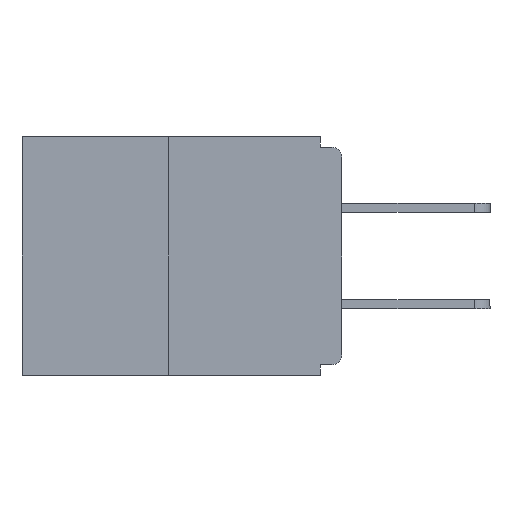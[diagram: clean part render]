
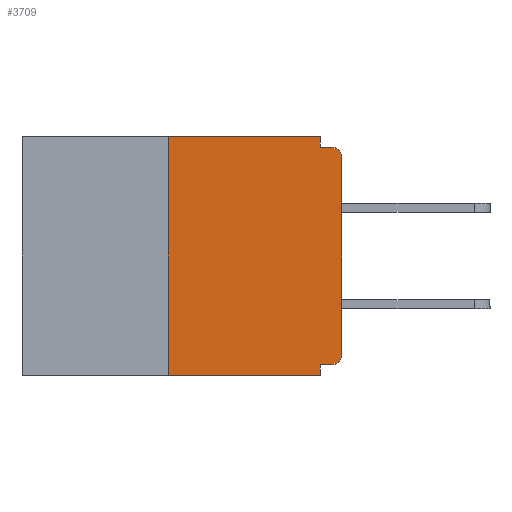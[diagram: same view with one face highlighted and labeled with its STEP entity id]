
A CAD part, left-side view. The second image highlights one B-rep face of the part: STEP entity #3709.
In plain terms, the highlighted planar face has unit normal (-1, 0, 0).
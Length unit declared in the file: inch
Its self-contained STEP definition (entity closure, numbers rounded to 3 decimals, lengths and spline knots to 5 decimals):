
#157 = CARTESIAN_POINT ( 'NONE',  ( 0., 0.015, -0.328 ) ) ;
#234 = AXIS2_PLACEMENT_3D ( 'NONE', #7054, #3540, #12680 ) ;
#275 = DIRECTION ( 'NONE',  ( 0., -1., 0. ) ) ;
#319 = VECTOR ( 'NONE', #4194, 39.37008 ) ;
#344 = VECTOR ( 'NONE', #21297, 39.37008 ) ;
#1178 = EDGE_CURVE ( 'NONE', #2732, #21505, #13912, .T. ) ;
#1779 = EDGE_CURVE ( 'NONE', #3134, #14864, #16443, .T. ) ;
#2047 = VERTEX_POINT ( 'NONE', #23496 ) ;
#2194 = DIRECTION ( 'NONE',  ( 0., 0., 1. ) ) ;
#2732 = VERTEX_POINT ( 'NONE', #4620 ) ;
#3070 = VECTOR ( 'NONE', #275, 39.37008 ) ;
#3134 = VERTEX_POINT ( 'NONE', #21408 ) ;
#3215 = CARTESIAN_POINT ( 'NONE',  ( 0., 0.031, -0.328 ) ) ;
#3540 = DIRECTION ( 'NONE',  ( -1., 0., 0. ) ) ;
#3709 = ADVANCED_FACE ( 'NONE', ( #12209 ), #12844, .F. ) ;
#3865 = CARTESIAN_POINT ( 'NONE',  ( 0., 0., -0.313 ) ) ;
#3996 = VECTOR ( 'NONE', #16205, 39.37008 ) ;
#4194 = DIRECTION ( 'NONE',  ( 0., 0., 1. ) ) ;
#4527 = EDGE_CURVE ( 'NONE', #3134, #17440, #16811, .T. ) ;
#4620 = CARTESIAN_POINT ( 'NONE',  ( 0., 0.031, 0. ) ) ;
#5381 = CIRCLE ( 'NONE', #9262, 0.015 ) ;
#5519 = ORIENTED_EDGE ( 'NONE', *, *, #21172, .F. ) ;
#5567 = CARTESIAN_POINT ( 'NONE',  ( 0., 0.031, 0. ) ) ;
#5667 = LINE ( 'NONE', #22235, #7079 ) ;
#6029 = VERTEX_POINT ( 'NONE', #3215 ) ;
#7054 = CARTESIAN_POINT ( 'NONE',  ( 0., 0.015, -0.313 ) ) ;
#7071 = CARTESIAN_POINT ( 'NONE',  ( 0., 0.46, 0. ) ) ;
#7079 = VECTOR ( 'NONE', #2194, 39.37008 ) ;
#7098 = ORIENTED_EDGE ( 'NONE', *, *, #11817, .T. ) ;
#7278 = DIRECTION ( 'NONE',  ( 1., 0., 0. ) ) ;
#8114 = EDGE_CURVE ( 'NONE', #17440, #2732, #13490, .T. ) ;
#8346 = ORIENTED_EDGE ( 'NONE', *, *, #1779, .T. ) ;
#8549 = LINE ( 'NONE', #21052, #344 ) ;
#8613 = VERTEX_POINT ( 'NONE', #157 ) ;
#9262 = AXIS2_PLACEMENT_3D ( 'NONE', #14672, #11026, #12928 ) ;
#9290 = CARTESIAN_POINT ( 'NONE',  ( 0., 0., -0.328 ) ) ;
#10149 = EDGE_CURVE ( 'NONE', #6029, #14864, #8549, .T. ) ;
#10155 = CARTESIAN_POINT ( 'NONE',  ( 0., 0.015, -0.015 ) ) ;
#10799 = CARTESIAN_POINT ( 'NONE',  ( 0., 0., -0.015 ) ) ;
#10881 = VECTOR ( 'NONE', #23419, 39.37008 ) ;
#10921 = CARTESIAN_POINT ( 'NONE',  ( 0., 0.031, -0.343 ) ) ;
#11026 = DIRECTION ( 'NONE',  ( -1., 0., 0. ) ) ;
#11188 = CARTESIAN_POINT ( 'NONE',  ( 0., 0.46, -0.343 ) ) ;
#11669 = CIRCLE ( 'NONE', #234, 0.015 ) ;
#11817 = EDGE_CURVE ( 'NONE', #8613, #19623, #11669, .T. ) ;
#11849 = DIRECTION ( 'NONE',  ( 0., 1., 0. ) ) ;
#12209 = FACE_OUTER_BOUND ( 'NONE', #12579, .T. ) ;
#12423 = ORIENTED_EDGE ( 'NONE', *, *, #15949, .F. ) ;
#12579 = EDGE_LOOP ( 'NONE', ( #21410, #13758, #8346, #14432, #5519, #7098, #16655, #15282, #12423, #14069 ) ) ;
#12680 = DIRECTION ( 'NONE',  ( 0., 0., -1. ) ) ;
#12844 = PLANE ( 'NONE',  #13531 ) ;
#12928 = DIRECTION ( 'NONE',  ( 0., 0., -1. ) ) ;
#13232 = VECTOR ( 'NONE', #23272, 39.37008 ) ;
#13490 = LINE ( 'NONE', #7071, #13232 ) ;
#13531 = AXIS2_PLACEMENT_3D ( 'NONE', #18147, #7278, #18231 ) ;
#13758 = ORIENTED_EDGE ( 'NONE', *, *, #4527, .F. ) ;
#13912 = LINE ( 'NONE', #5567, #3996 ) ;
#14069 = ORIENTED_EDGE ( 'NONE', *, *, #1178, .F. ) ;
#14351 = LINE ( 'NONE', #9290, #14944 ) ;
#14432 = ORIENTED_EDGE ( 'NONE', *, *, #10149, .F. ) ;
#14672 = CARTESIAN_POINT ( 'NONE',  ( 0., 0.015, -0.03 ) ) ;
#14864 = VERTEX_POINT ( 'NONE', #10921 ) ;
#14944 = VECTOR ( 'NONE', #11849, 39.37008 ) ;
#15082 = CARTESIAN_POINT ( 'NONE',  ( 0., 0.25, 0. ) ) ;
#15282 = ORIENTED_EDGE ( 'NONE', *, *, #19414, .T. ) ;
#15949 = EDGE_CURVE ( 'NONE', #21505, #22484, #18247, .T. ) ;
#16205 = DIRECTION ( 'NONE',  ( 0., 0., -1. ) ) ;
#16421 = CARTESIAN_POINT ( 'NONE',  ( 0., 0.031, -0.015 ) ) ;
#16443 = LINE ( 'NONE', #11188, #3070 ) ;
#16655 = ORIENTED_EDGE ( 'NONE', *, *, #19569, .T. ) ;
#16753 = CARTESIAN_POINT ( 'NONE',  ( 0., 0.25, 0. ) ) ;
#16811 = LINE ( 'NONE', #15082, #319 ) ;
#17440 = VERTEX_POINT ( 'NONE', #16753 ) ;
#18147 = CARTESIAN_POINT ( 'NONE',  ( 0., 0.46, 0. ) ) ;
#18231 = DIRECTION ( 'NONE',  ( 0., 0., -1. ) ) ;
#18247 = LINE ( 'NONE', #10799, #10881 ) ;
#19414 = EDGE_CURVE ( 'NONE', #2047, #22484, #5381, .T. ) ;
#19569 = EDGE_CURVE ( 'NONE', #19623, #2047, #5667, .T. ) ;
#19623 = VERTEX_POINT ( 'NONE', #3865 ) ;
#21052 = CARTESIAN_POINT ( 'NONE',  ( 0., 0.031, -0.343 ) ) ;
#21172 = EDGE_CURVE ( 'NONE', #8613, #6029, #14351, .T. ) ;
#21297 = DIRECTION ( 'NONE',  ( 0., 0., -1. ) ) ;
#21408 = CARTESIAN_POINT ( 'NONE',  ( 0., 0.25, -0.343 ) ) ;
#21410 = ORIENTED_EDGE ( 'NONE', *, *, #8114, .F. ) ;
#21505 = VERTEX_POINT ( 'NONE', #16421 ) ;
#22235 = CARTESIAN_POINT ( 'NONE',  ( 0., 0., 0. ) ) ;
#22484 = VERTEX_POINT ( 'NONE', #10155 ) ;
#23272 = DIRECTION ( 'NONE',  ( 0., -1., 0. ) ) ;
#23419 = DIRECTION ( 'NONE',  ( 0., -1., 0. ) ) ;
#23496 = CARTESIAN_POINT ( 'NONE',  ( 0., 0., -0.03 ) ) ;
